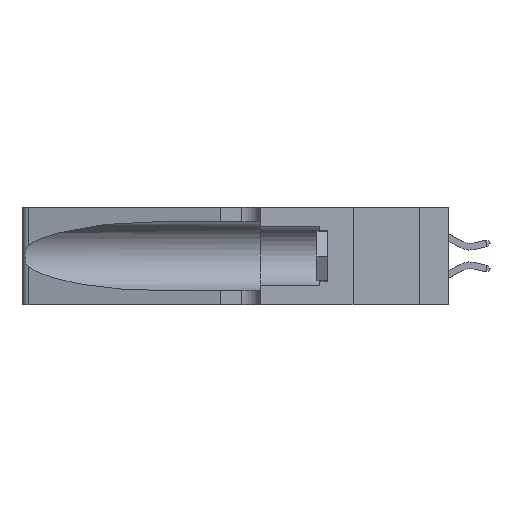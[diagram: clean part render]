
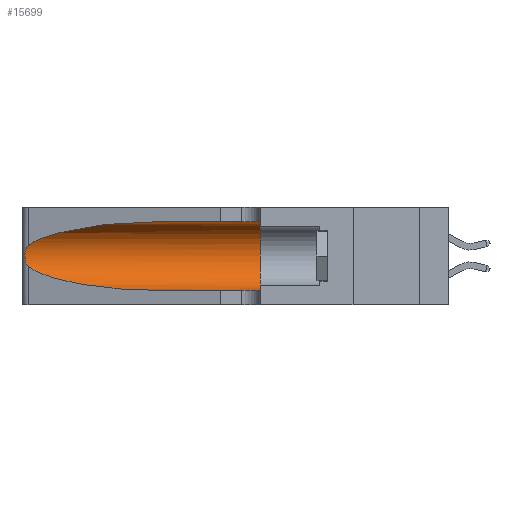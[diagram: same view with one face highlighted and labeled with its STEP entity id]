
A CAD part, left-side view. The second image highlights one B-rep face of the part: STEP entity #15699.
In plain terms, the highlighted cylindrical face has radius 3.308 mm (diameter 6.617 mm), a partial arc.
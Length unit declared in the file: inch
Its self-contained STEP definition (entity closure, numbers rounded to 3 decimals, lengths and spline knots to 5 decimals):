
#1219 = EDGE_CURVE ( 'NONE', #8215, #22637, #9935, .T. ) ;
#2484 = CARTESIAN_POINT ( 'NONE',  ( 0.25856, 1.23593, 0.16098 ) ) ;
#2962 = VERTEX_POINT ( 'NONE', #6936 ) ;
#3176 = EDGE_LOOP ( 'NONE', ( #6828, #22176, #37414, #8643, #16442, #3626 ) ) ;
#3303 = CARTESIAN_POINT ( 'NONE',  ( 0.18966, 0.96281, 0.31525 ) ) ;
#3626 = ORIENTED_EDGE ( 'NONE', *, *, #33512, .F. ) ;
#4498 = CARTESIAN_POINT ( 'NONE',  ( 0.1305, 1.61858, 0.05475 ) ) ;
#5105 = CARTESIAN_POINT ( 'NONE',  ( 0.25487, 1.22718, 0.14631 ) ) ;
#5133 = CARTESIAN_POINT ( 'NONE',  ( 0.1305, 1.61858, 0.31525 ) ) ;
#5237 = CARTESIAN_POINT ( 'NONE',  ( 0.1305, 0.35, 0.185 ) ) ;
#5338 = CARTESIAN_POINT ( 'NONE',  ( 0.25555, 1.22994, 0.2215 ) ) ;
#5452 = CARTESIAN_POINT ( 'NONE',  ( 0.25639, 1.23186, 0.15144 ) ) ;
#6259 = CARTESIAN_POINT ( 'NONE',  ( 0.2373, 1.15595, 0.28018 ) ) ;
#6419 = CARTESIAN_POINT ( 'NONE',  ( 0.1305, 0.72297, 0.31525 ) ) ;
#6828 = ORIENTED_EDGE ( 'NONE', *, *, #11061, .T. ) ;
#6936 = CARTESIAN_POINT ( 'NONE',  ( 0.1305, 0.35, 0.31525 ) ) ;
#7537 = EDGE_CURVE ( 'NONE', #22637, #35708, #33409, .T. ) ;
#8115 = VECTOR ( 'NONE', #22429, 39.37008 ) ;
#8154 = DIRECTION ( 'NONE',  ( 0., 0., 1. ) ) ;
#8215 = VERTEX_POINT ( 'NONE', #5105 ) ;
#8360 = CARTESIAN_POINT ( 'NONE',  ( 0.25487, 1.22718, 0.14631 ) ) ;
#8643 = ORIENTED_EDGE ( 'NONE', *, *, #7537, .T. ) ;
#9200 = AXIS2_PLACEMENT_3D ( 'NONE', #12363, #32396, #29496 ) ;
#9935 =( BOUNDED_CURVE ( )  B_SPLINE_CURVE ( 3, ( #33692, #27948, #30822, #16633 ),
 .UNSPECIFIED., .F., .T. ) 
 B_SPLINE_CURVE_WITH_KNOTS ( ( 4, 4 ),
 ( 3.44316, 4.71239 ),
 .UNSPECIFIED. ) 
 CURVE ( )  GEOMETRIC_REPRESENTATION_ITEM ( )  RATIONAL_B_SPLINE_CURVE ( ( 1., 0.87, 0.87, 1. ) ) 
 REPRESENTATION_ITEM ( '' )  );
#11061 = EDGE_CURVE ( 'NONE', #16441, #26076, #20576, .T. ) ;
#11186 = CARTESIAN_POINT ( 'NONE',  ( 0.25639, 1.23184, 0.21858 ) ) ;
#11681 = CARTESIAN_POINT ( 'NONE',  ( 0.1305, 0.72297, 0.05475 ) ) ;
#12363 = CARTESIAN_POINT ( 'NONE',  ( 0.1305, 1.61858, 0.185 ) ) ;
#14142 = CARTESIAN_POINT ( 'NONE',  ( 0.25854, 1.2359, 0.20912 ) ) ;
#15699 = ADVANCED_FACE ( 'NONE', ( #22860 ), #37195, .F. ) ;
#16441 = VERTEX_POINT ( 'NONE', #6419 ) ;
#16442 = ORIENTED_EDGE ( 'NONE', *, *, #17375, .F. ) ;
#16633 = CARTESIAN_POINT ( 'NONE',  ( 0.1305, 0.72297, 0.05475 ) ) ;
#17060 = CARTESIAN_POINT ( 'NONE',  ( 0.26075, 1.23896, 0.19203 ) ) ;
#17375 = EDGE_CURVE ( 'NONE', #2962, #35708, #22782, .T. ) ;
#18254 = VECTOR ( 'NONE', #36093, 39.37008 ) ;
#19911 = CARTESIAN_POINT ( 'NONE',  ( 0.26017, 1.23833, 0.17102 ) ) ;
#20576 =( BOUNDED_CURVE ( )  B_SPLINE_CURVE ( 3, ( #23540, #3303, #6259, #26393 ),
 .UNSPECIFIED., .F., .F. ) 
 B_SPLINE_CURVE_WITH_KNOTS ( ( 4, 4 ),
 ( 1.5708, 2.84003 ),
 .UNSPECIFIED. ) 
 CURVE ( )  GEOMETRIC_REPRESENTATION_ITEM ( )  RATIONAL_B_SPLINE_CURVE ( ( 1., 0.87, 0.87, 1. ) ) 
 REPRESENTATION_ITEM ( '' )  );
#22176 = ORIENTED_EDGE ( 'NONE', *, *, #22558, .T. ) ;
#22429 = DIRECTION ( 'NONE',  ( 0., -1., 0. ) ) ;
#22558 = EDGE_CURVE ( 'NONE', #26076, #8215, #24446, .T. ) ;
#22637 = VERTEX_POINT ( 'NONE', #11681 ) ;
#22736 = CARTESIAN_POINT ( 'NONE',  ( 0.25789, 1.23486, 0.15765 ) ) ;
#22782 = CIRCLE ( 'NONE', #33790, 0.13025 ) ;
#22860 = FACE_OUTER_BOUND ( 'NONE', #3176, .T. ) ;
#23540 = CARTESIAN_POINT ( 'NONE',  ( 0.1305, 0.72297, 0.31525 ) ) ;
#24446 = B_SPLINE_CURVE_WITH_KNOTS ( 'NONE', 3,
 ( #25466, #5338, #11186, #31238, #14142, #34117, #17060, #37014, #19911, #2484, #22736, #5452, #25596, #8360 ),
 .UNSPECIFIED., .F., .F.,
 ( 4, 2, 2, 2, 2, 2, 4 ),
 ( 0., 0.00027, 0.00053, 0.00107, 0.0016, 0.00187, 0.00214 ),
 .UNSPECIFIED. ) ;
#24979 = CARTESIAN_POINT ( 'NONE',  ( 0.1305, 0.35, 0.05475 ) ) ;
#25374 = DIRECTION ( 'NONE',  ( 0., 1., 0. ) ) ;
#25466 = CARTESIAN_POINT ( 'NONE',  ( 0.25487, 1.22718, 0.22369 ) ) ;
#25596 = CARTESIAN_POINT ( 'NONE',  ( 0.25555, 1.22993, 0.14849 ) ) ;
#26076 = VERTEX_POINT ( 'NONE', #26077 ) ;
#26077 = CARTESIAN_POINT ( 'NONE',  ( 0.25487, 1.22718, 0.22369 ) ) ;
#26393 = CARTESIAN_POINT ( 'NONE',  ( 0.25487, 1.22718, 0.22369 ) ) ;
#27948 = CARTESIAN_POINT ( 'NONE',  ( 0.2373, 1.15595, 0.08982 ) ) ;
#29496 = DIRECTION ( 'NONE',  ( 0., 0., -1. ) ) ;
#30822 = CARTESIAN_POINT ( 'NONE',  ( 0.18966, 0.96281, 0.05475 ) ) ;
#31043 = LINE ( 'NONE', #5133, #8115 ) ;
#31238 = CARTESIAN_POINT ( 'NONE',  ( 0.25787, 1.23484, 0.2124 ) ) ;
#32396 = DIRECTION ( 'NONE',  ( 0., -1., 0. ) ) ;
#33409 = LINE ( 'NONE', #4498, #18254 ) ;
#33512 = EDGE_CURVE ( 'NONE', #16441, #2962, #31043, .T. ) ;
#33692 = CARTESIAN_POINT ( 'NONE',  ( 0.25487, 1.22718, 0.14631 ) ) ;
#33790 = AXIS2_PLACEMENT_3D ( 'NONE', #5237, #25374, #8154 ) ;
#34117 = CARTESIAN_POINT ( 'NONE',  ( 0.26018, 1.23835, 0.19895 ) ) ;
#35708 = VERTEX_POINT ( 'NONE', #24979 ) ;
#36093 = DIRECTION ( 'NONE',  ( 0., -1., 0. ) ) ;
#37014 = CARTESIAN_POINT ( 'NONE',  ( 0.26075, 1.23896, 0.178 ) ) ;
#37195 = CYLINDRICAL_SURFACE ( 'NONE', #9200, 0.13025 ) ;
#37414 = ORIENTED_EDGE ( 'NONE', *, *, #1219, .T. ) ;
